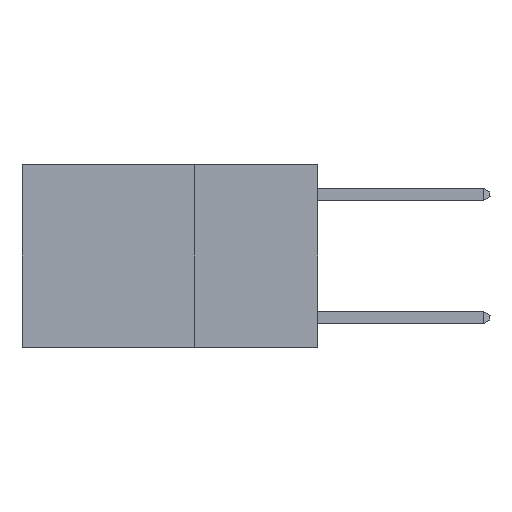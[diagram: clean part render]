
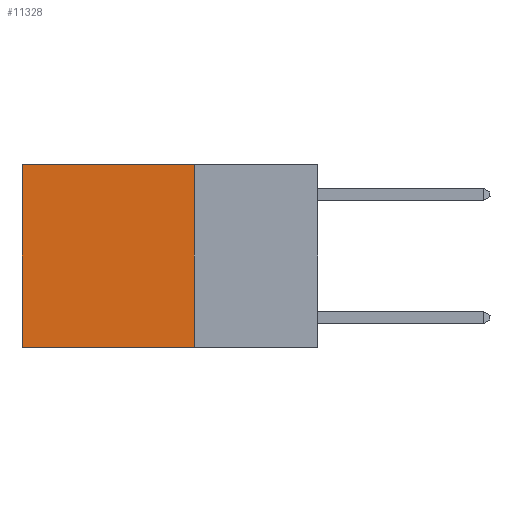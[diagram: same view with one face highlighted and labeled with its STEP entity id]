
A CAD part, left-side view. The second image highlights one B-rep face of the part: STEP entity #11328.
In plain terms, the highlighted planar face has unit normal (-1, 0, 0).
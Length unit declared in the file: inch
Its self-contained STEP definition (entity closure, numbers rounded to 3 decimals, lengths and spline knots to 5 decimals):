
#79 = VERTEX_POINT ( 'NONE', #9906 ) ;
#209 = DIRECTION ( 'NONE',  ( 0., 0., -1. ) ) ;
#709 = VECTOR ( 'NONE', #1783, 39.37008 ) ;
#1337 = EDGE_CURVE ( 'NONE', #79, #9614, #3232, .T. ) ;
#1542 = ORIENTED_EDGE ( 'NONE', *, *, #5237, .F. ) ;
#1776 = VECTOR ( 'NONE', #8691, 39.37008 ) ;
#1783 = DIRECTION ( 'NONE',  ( 0., 1., 0. ) ) ;
#2411 = CARTESIAN_POINT ( 'NONE',  ( 0.2625, 0.25, 0. ) ) ;
#2725 = EDGE_CURVE ( 'NONE', #2948, #9614, #11072, .T. ) ;
#2948 = VERTEX_POINT ( 'NONE', #7970 ) ;
#3232 = LINE ( 'NONE', #7583, #11086 ) ;
#3287 = ORIENTED_EDGE ( 'NONE', *, *, #2725, .T. ) ;
#5153 = CARTESIAN_POINT ( 'NONE',  ( 0.2625, 0.25, 0. ) ) ;
#5201 = LINE ( 'NONE', #5153, #1776 ) ;
#5237 = EDGE_CURVE ( 'NONE', #7055, #79, #5201, .T. ) ;
#5404 = ORIENTED_EDGE ( 'NONE', *, *, #8852, .T. ) ;
#5493 = ORIENTED_EDGE ( 'NONE', *, *, #1337, .F. ) ;
#6768 = DIRECTION ( 'NONE',  ( 0., 1., 0. ) ) ;
#7055 = VERTEX_POINT ( 'NONE', #2411 ) ;
#7312 = CARTESIAN_POINT ( 'NONE',  ( 0.2625, 0.6, 0. ) ) ;
#7583 = CARTESIAN_POINT ( 'NONE',  ( 0.2625, 0.25, -0.37 ) ) ;
#7900 = CARTESIAN_POINT ( 'NONE',  ( 0.2625, 0.6, -0.37 ) ) ;
#7970 = CARTESIAN_POINT ( 'NONE',  ( 0.2625, 0.6, 0. ) ) ;
#8691 = DIRECTION ( 'NONE',  ( 0., 0., -1. ) ) ;
#8852 = EDGE_CURVE ( 'NONE', #7055, #2948, #9710, .T. ) ;
#8905 = PLANE ( 'NONE',  #10659 ) ;
#8970 = DIRECTION ( 'NONE',  ( 1., 0., 0. ) ) ;
#9614 = VERTEX_POINT ( 'NONE', #7900 ) ;
#9655 = CARTESIAN_POINT ( 'NONE',  ( 0.2625, 0.25, 0. ) ) ;
#9699 = CARTESIAN_POINT ( 'NONE',  ( 0.2625, 0.25, 0. ) ) ;
#9710 = LINE ( 'NONE', #9655, #709 ) ;
#9819 = FACE_OUTER_BOUND ( 'NONE', #10756, .T. ) ;
#9906 = CARTESIAN_POINT ( 'NONE',  ( 0.2625, 0.25, -0.37 ) ) ;
#9916 = DIRECTION ( 'NONE',  ( 0., 0., -1. ) ) ;
#10431 = VECTOR ( 'NONE', #9916, 39.37008 ) ;
#10659 = AXIS2_PLACEMENT_3D ( 'NONE', #9699, #8970, #209 ) ;
#10756 = EDGE_LOOP ( 'NONE', ( #3287, #5493, #1542, #5404 ) ) ;
#11072 = LINE ( 'NONE', #7312, #10431 ) ;
#11086 = VECTOR ( 'NONE', #6768, 39.37008 ) ;
#11328 = ADVANCED_FACE ( 'NONE', ( #9819 ), #8905, .F. ) ;
